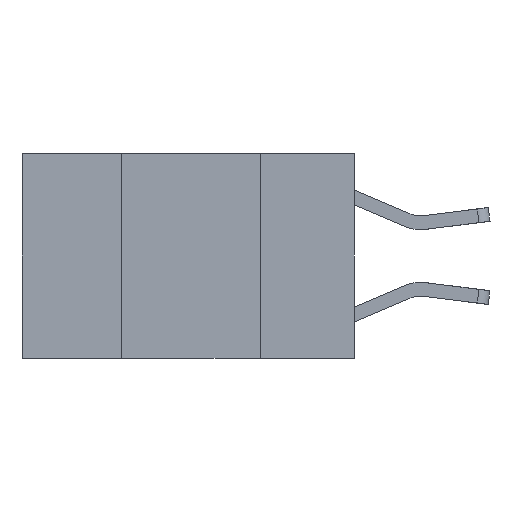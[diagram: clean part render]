
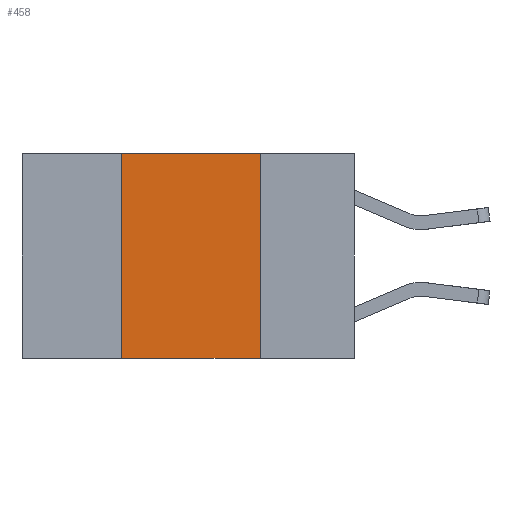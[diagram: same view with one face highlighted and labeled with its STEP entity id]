
A CAD part, left-side view. The second image highlights one B-rep face of the part: STEP entity #458.
In plain terms, the highlighted planar face has unit normal (-1, 0, 0).
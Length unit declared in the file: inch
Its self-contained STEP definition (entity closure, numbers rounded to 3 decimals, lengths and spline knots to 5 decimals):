
#214 = ORIENTED_EDGE ( 'NONE', *, *, #8526, .F. ) ;
#458 = ADVANCED_FACE ( 'NONE', ( #7551 ), #7909, .F. ) ;
#1073 = DIRECTION ( 'NONE',  ( 0., 0., -1. ) ) ;
#1382 = LINE ( 'NONE', #6214, #8898 ) ;
#1569 = VECTOR ( 'NONE', #4939, 39.37008 ) ;
#1616 = DIRECTION ( 'NONE',  ( 0., 0., -1. ) ) ;
#1827 = DIRECTION ( 'NONE',  ( 0., -1., 0. ) ) ;
#1891 = VERTEX_POINT ( 'NONE', #8449 ) ;
#2039 = DIRECTION ( 'NONE',  ( 1., 0., 0. ) ) ;
#2468 = EDGE_CURVE ( 'NONE', #8248, #7450, #9286, .T. ) ;
#2839 = AXIS2_PLACEMENT_3D ( 'NONE', #6515, #2039, #1073 ) ;
#3100 = ORIENTED_EDGE ( 'NONE', *, *, #2468, .F. ) ;
#4241 = ORIENTED_EDGE ( 'NONE', *, *, #4648, .T. ) ;
#4600 = LINE ( 'NONE', #7656, #7784 ) ;
#4648 = EDGE_CURVE ( 'NONE', #1891, #6228, #1382, .T. ) ;
#4762 = DIRECTION ( 'NONE',  ( 0., 0., 1. ) ) ;
#4939 = DIRECTION ( 'NONE',  ( 0., -1., 0. ) ) ;
#5059 = ORIENTED_EDGE ( 'NONE', *, *, #5629, .F. ) ;
#5064 = CARTESIAN_POINT ( 'NONE',  ( 0., 0.42, 0. ) ) ;
#5489 = EDGE_LOOP ( 'NONE', ( #214, #3100, #5059, #4241 ) ) ;
#5520 = CARTESIAN_POINT ( 'NONE',  ( 0., 0.17, -0.37 ) ) ;
#5629 = EDGE_CURVE ( 'NONE', #1891, #8248, #4600, .T. ) ;
#5679 = LINE ( 'NONE', #6745, #9045 ) ;
#6214 = CARTESIAN_POINT ( 'NONE',  ( 0., 0.6, -0.37 ) ) ;
#6228 = VERTEX_POINT ( 'NONE', #5520 ) ;
#6515 = CARTESIAN_POINT ( 'NONE',  ( 0., 0.6, 0. ) ) ;
#6745 = CARTESIAN_POINT ( 'NONE',  ( 0., 0.17, 0. ) ) ;
#7450 = VERTEX_POINT ( 'NONE', #7977 ) ;
#7551 = FACE_OUTER_BOUND ( 'NONE', #5489, .T. ) ;
#7656 = CARTESIAN_POINT ( 'NONE',  ( 0., 0.42, 0. ) ) ;
#7784 = VECTOR ( 'NONE', #4762, 39.37008 ) ;
#7909 = PLANE ( 'NONE',  #2839 ) ;
#7977 = CARTESIAN_POINT ( 'NONE',  ( 0., 0.17, 0. ) ) ;
#8248 = VERTEX_POINT ( 'NONE', #5064 ) ;
#8449 = CARTESIAN_POINT ( 'NONE',  ( 0., 0.42, -0.37 ) ) ;
#8526 = EDGE_CURVE ( 'NONE', #7450, #6228, #5679, .T. ) ;
#8898 = VECTOR ( 'NONE', #1827, 39.37008 ) ;
#9045 = VECTOR ( 'NONE', #1616, 39.37008 ) ;
#9193 = CARTESIAN_POINT ( 'NONE',  ( 0., 0.6, 0. ) ) ;
#9286 = LINE ( 'NONE', #9193, #1569 ) ;
